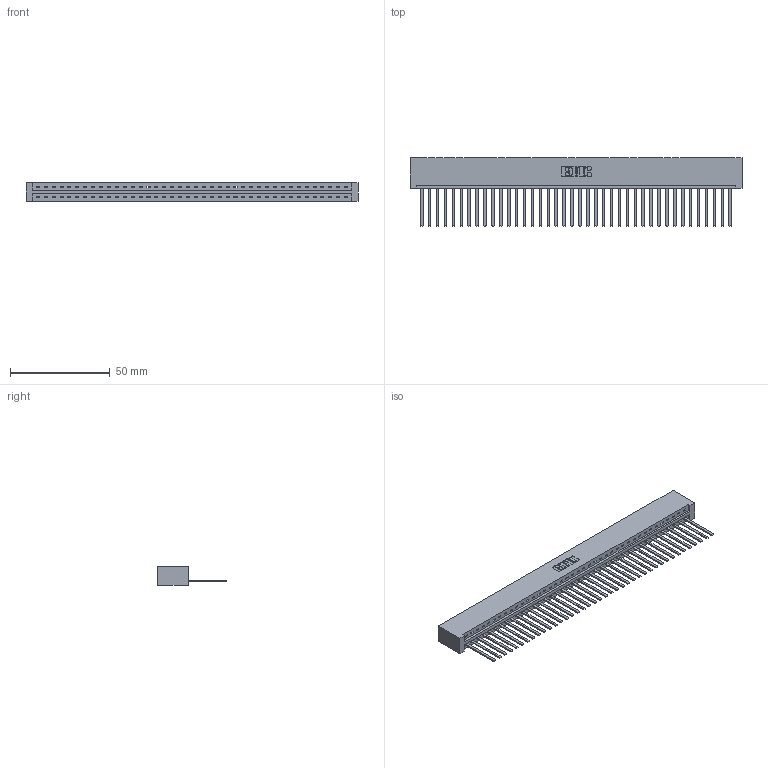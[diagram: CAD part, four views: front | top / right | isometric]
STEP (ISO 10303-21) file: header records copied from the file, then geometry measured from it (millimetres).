
FILE_DESCRIPTION (( 'STEP AP203' ), '1' );
FILE_NAME ('387-040-544-101.STEP', '2018-09-19T16:35:18', ( '' ), ( '' ), 'SwSTEP 2.0', 'SolidWorks 2016', '' );
FILE_SCHEMA (( 'CONFIG_CONTROL_DESIGN' ));
Length unit declared in the file: inch
Products named in the file (3): 337 Part_No Mounting Lugs; 345-292-001_345-293-144; 387-040-544-101
Assembly tree (41 placements, depth 2):
  387-040-544-101
    337 Part_No Mounting Lugs
    345-292-001_345-293-144  x40
Bounding box: 166.37 x 34.3 x 9.4 mm (x, y, z)
Volume: 18468.3 mm3; surface area: 20578.5 mm2
Topology: 41 solids, 41 shells, 2346 faces, 7087 edges, 4670 vertices
Faces by surface type: plane 1746, cylinder 600
Entity records: 29531 total; most frequent: CARTESIAN_POINT 5150, ORIENTED_EDGE 5126, DIRECTION 4327, EDGE_CURVE 2563, VECTOR 2447, LINE 2447, VERTEX_POINT 1706, AXIS2_PLACEMENT_3D 940
